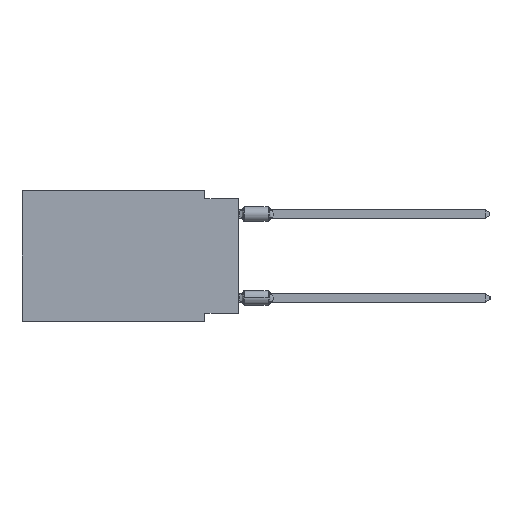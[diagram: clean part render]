
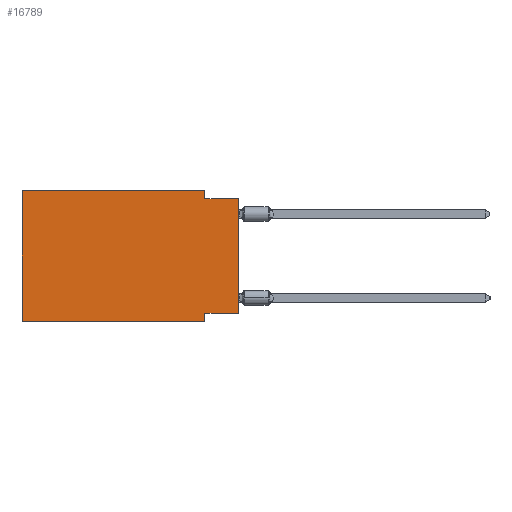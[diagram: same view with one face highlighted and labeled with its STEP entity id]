
A CAD part, left-side view. The second image highlights one B-rep face of the part: STEP entity #16789.
In plain terms, the highlighted planar face has unit normal (-1, 0, 0).
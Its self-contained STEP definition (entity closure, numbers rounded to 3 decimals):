
#1012 = LINE ( 'NONE', #17122, #37422 ) ;
#1878 = VERTEX_POINT ( 'NONE', #5259 ) ;
#2517 = ORIENTED_EDGE ( 'NONE', *, *, #44991, .T. ) ;
#2757 = CARTESIAN_POINT ( 'NONE',  ( 0., 0., -0.635 ) ) ;
#2890 = ORIENTED_EDGE ( 'NONE', *, *, #35325, .F. ) ;
#3663 = VERTEX_POINT ( 'NONE', #51395 ) ;
#4725 = ORIENTED_EDGE ( 'NONE', *, *, #14250, .F. ) ;
#5259 = CARTESIAN_POINT ( 'NONE',  ( 0., 16.383, 0. ) ) ;
#5520 = CARTESIAN_POINT ( 'NONE',  ( 0., 0., 0. ) ) ;
#5609 = CARTESIAN_POINT ( 'NONE',  ( 0., 2.54, -9.271 ) ) ;
#7665 = VERTEX_POINT ( 'NONE', #44027 ) ;
#8952 = DIRECTION ( 'NONE',  ( 0., 1., 0. ) ) ;
#9209 = DIRECTION ( 'NONE',  ( 0., 0., -1. ) ) ;
#12260 = DIRECTION ( 'NONE',  ( 0., -1., 0. ) ) ;
#12571 = CARTESIAN_POINT ( 'NONE',  ( 0., 16.383, -9.906 ) ) ;
#13763 = VERTEX_POINT ( 'NONE', #25397 ) ;
#13985 = EDGE_CURVE ( 'NONE', #27521, #1878, #46490, .T. ) ;
#14074 = PLANE ( 'NONE',  #31598 ) ;
#14250 = EDGE_CURVE ( 'NONE', #16176, #33121, #29286, .T. ) ;
#14593 = DIRECTION ( 'NONE',  ( 0., 0., -1. ) ) ;
#15075 = DIRECTION ( 'NONE',  ( 0., 0., 1. ) ) ;
#15928 = LINE ( 'NONE', #44969, #18299 ) ;
#16176 = VERTEX_POINT ( 'NONE', #5609 ) ;
#16771 = CARTESIAN_POINT ( 'NONE',  ( 0., 2.54, -0.635 ) ) ;
#16789 = ADVANCED_FACE ( 'NONE', ( #21984 ), #14074, .F. ) ;
#17122 = CARTESIAN_POINT ( 'NONE',  ( 0., 0., -9.271 ) ) ;
#17137 = DIRECTION ( 'NONE',  ( 0., 0., 1. ) ) ;
#18299 = VECTOR ( 'NONE', #12260, 1000. ) ;
#18865 = DIRECTION ( 'NONE',  ( 0., -1., 0. ) ) ;
#19231 = ORIENTED_EDGE ( 'NONE', *, *, #13985, .F. ) ;
#19620 = VECTOR ( 'NONE', #17137, 1000. ) ;
#21631 = CARTESIAN_POINT ( 'NONE',  ( 0., 2.54, -9.906 ) ) ;
#21984 = FACE_OUTER_BOUND ( 'NONE', #38581, .T. ) ;
#22211 = VECTOR ( 'NONE', #18865, 1000. ) ;
#24275 = DIRECTION ( 'NONE',  ( 0., 0., -1. ) ) ;
#25397 = CARTESIAN_POINT ( 'NONE',  ( 0., 0., -9.271 ) ) ;
#26217 = ORIENTED_EDGE ( 'NONE', *, *, #44056, .T. ) ;
#26350 = VECTOR ( 'NONE', #15075, 1000. ) ;
#27521 = VERTEX_POINT ( 'NONE', #35851 ) ;
#28743 = LINE ( 'NONE', #39846, #31811 ) ;
#28833 = EDGE_CURVE ( 'NONE', #13763, #16176, #1012, .T. ) ;
#29286 = LINE ( 'NONE', #21631, #36586 ) ;
#31598 = AXIS2_PLACEMENT_3D ( 'NONE', #34411, #50246, #14593 ) ;
#31811 = VECTOR ( 'NONE', #24275, 1000. ) ;
#33121 = VERTEX_POINT ( 'NONE', #51590 ) ;
#34411 = CARTESIAN_POINT ( 'NONE',  ( 0., 16.383, 0. ) ) ;
#35325 = EDGE_CURVE ( 'NONE', #3663, #48209, #28743, .T. ) ;
#35851 = CARTESIAN_POINT ( 'NONE',  ( 0., 16.383, -9.906 ) ) ;
#36348 = DIRECTION ( 'NONE',  ( 0., -1., 0. ) ) ;
#36586 = VECTOR ( 'NONE', #9209, 1000. ) ;
#37083 = EDGE_CURVE ( 'NONE', #1878, #3663, #15928, .T. ) ;
#37422 = VECTOR ( 'NONE', #8952, 1000. ) ;
#38581 = EDGE_LOOP ( 'NONE', ( #2517, #52142, #2890, #39108, #19231, #26217, #4725, #41811 ) ) ;
#38934 = LINE ( 'NONE', #2757, #22211 ) ;
#39108 = ORIENTED_EDGE ( 'NONE', *, *, #37083, .F. ) ;
#39846 = CARTESIAN_POINT ( 'NONE',  ( 0., 2.54, 0. ) ) ;
#41690 = LINE ( 'NONE', #5520, #19620 ) ;
#41811 = ORIENTED_EDGE ( 'NONE', *, *, #28833, .F. ) ;
#42803 = CARTESIAN_POINT ( 'NONE',  ( 0., 16.383, 0. ) ) ;
#44027 = CARTESIAN_POINT ( 'NONE',  ( 0., 0., -0.635 ) ) ;
#44056 = EDGE_CURVE ( 'NONE', #27521, #33121, #48742, .T. ) ;
#44969 = CARTESIAN_POINT ( 'NONE',  ( 0., 16.383, 0. ) ) ;
#44991 = EDGE_CURVE ( 'NONE', #13763, #7665, #41690, .T. ) ;
#46490 = LINE ( 'NONE', #42803, #26350 ) ;
#47286 = EDGE_CURVE ( 'NONE', #48209, #7665, #38934, .T. ) ;
#47446 = VECTOR ( 'NONE', #36348, 1000. ) ;
#48209 = VERTEX_POINT ( 'NONE', #16771 ) ;
#48742 = LINE ( 'NONE', #12571, #47446 ) ;
#50246 = DIRECTION ( 'NONE',  ( 1., 0., 0. ) ) ;
#51395 = CARTESIAN_POINT ( 'NONE',  ( 0., 2.54, 0. ) ) ;
#51590 = CARTESIAN_POINT ( 'NONE',  ( 0., 2.54, -9.906 ) ) ;
#52142 = ORIENTED_EDGE ( 'NONE', *, *, #47286, .F. ) ;
